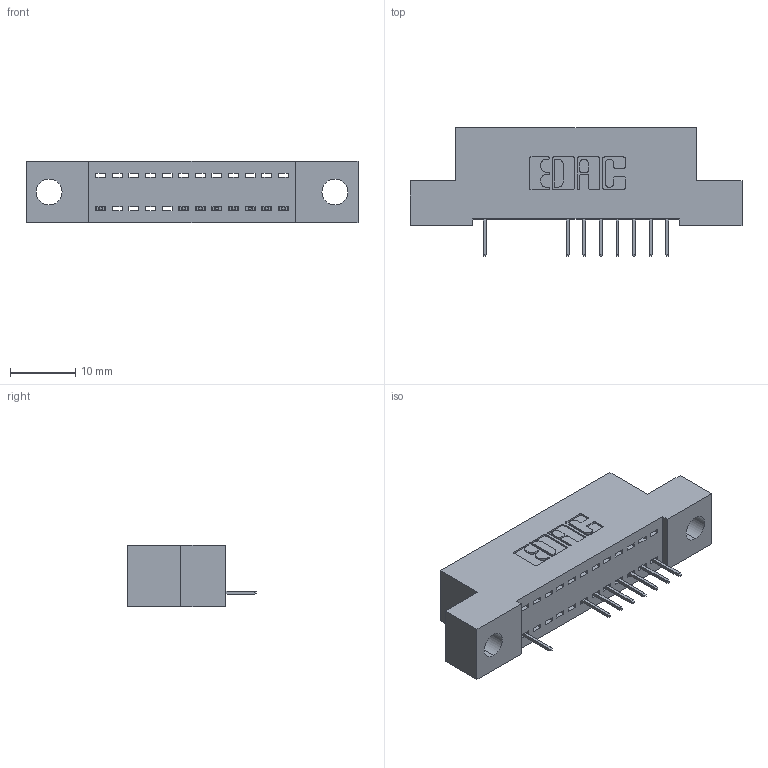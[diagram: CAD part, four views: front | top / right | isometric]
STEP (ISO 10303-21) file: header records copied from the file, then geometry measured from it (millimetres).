
FILE_DESCRIPTION (( 'STEP AP203' ), '1' );
FILE_NAME ('392-012-524-104.STEP', '2018-08-14T21:56:00', ( '' ), ( '' ), 'SwSTEP 2.0', 'SolidWorks 2016', '' );
FILE_SCHEMA (( 'CONFIG_CONTROL_DESIGN' ));
Length unit declared in the file: inch
Products named in the file (3): 392-012-524-104; 342 Part_.156 TH; 345-292-001_345-293-124
Assembly tree (9 placements, depth 2):
  392-012-524-104
    342 Part_.156 TH
    345-292-001_345-293-124  x8
Bounding box: 50.8 x 19.69 x 9.4 mm (x, y, z)
Volume: 4179.3 mm3; surface area: 5060.5 mm2
Topology: 9 solids, 9 shells, 654 faces, 1907 edges, 1238 vertices
Faces by surface type: plane 498, cylinder 156
Entity records: 11033 total; most frequent: CARTESIAN_POINT 1930, ORIENTED_EDGE 1882, DIRECTION 1685, EDGE_CURVE 941, LINE 817, VECTOR 817, VERTEX_POINT 622, AXIS2_PLACEMENT_3D 434
